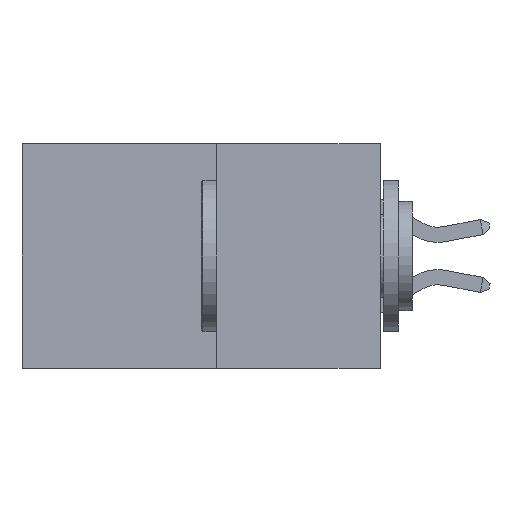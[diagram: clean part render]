
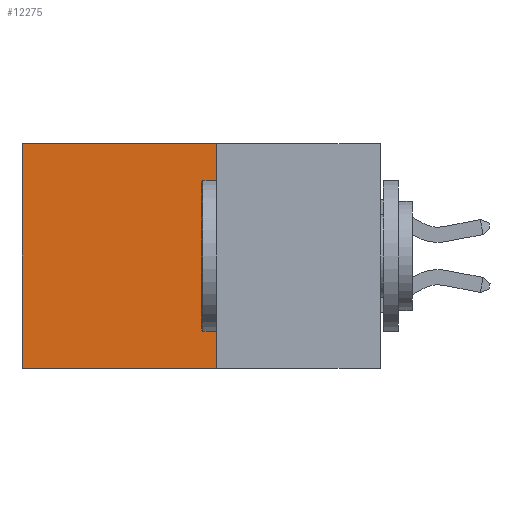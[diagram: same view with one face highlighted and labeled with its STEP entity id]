
A CAD part, left-side view. The second image highlights one B-rep face of the part: STEP entity #12275.
In plain terms, the highlighted planar face has unit normal (-1, 0, 0).
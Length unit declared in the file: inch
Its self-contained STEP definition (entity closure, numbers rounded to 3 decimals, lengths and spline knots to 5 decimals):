
#69 = ORIENTED_EDGE ( 'NONE', *, *, #7049, .F. ) ;
#188 = CARTESIAN_POINT ( 'NONE',  ( 0.277, 0.59, 0. ) ) ;
#551 = FACE_OUTER_BOUND ( 'NONE', #9237, .T. ) ;
#768 = DIRECTION ( 'NONE',  ( 0., 0., -1. ) ) ;
#949 = ORIENTED_EDGE ( 'NONE', *, *, #8611, .T. ) ;
#1112 = LINE ( 'NONE', #6383, #6055 ) ;
#1419 = DIRECTION ( 'NONE',  ( 0., 1., 0. ) ) ;
#1436 = CARTESIAN_POINT ( 'NONE',  ( 0.277, 0.27, 0. ) ) ;
#1829 = DIRECTION ( 'NONE',  ( 1., 0., 0. ) ) ;
#1876 = CARTESIAN_POINT ( 'NONE',  ( 0.277, 0.27, -0.37 ) ) ;
#2864 = PLANE ( 'NONE',  #3620 ) ;
#2878 = CARTESIAN_POINT ( 'NONE',  ( 0.277, 0.59, -0.37 ) ) ;
#2909 = VERTEX_POINT ( 'NONE', #2934 ) ;
#2934 = CARTESIAN_POINT ( 'NONE',  ( 0.277, 0.27, 0. ) ) ;
#3247 = EDGE_CURVE ( 'NONE', #4956, #11204, #1112, .T. ) ;
#3551 = VERTEX_POINT ( 'NONE', #188 ) ;
#3620 = AXIS2_PLACEMENT_3D ( 'NONE', #1876, #1829, #3857 ) ;
#3857 = DIRECTION ( 'NONE',  ( 0., 0., -1. ) ) ;
#4673 = ORIENTED_EDGE ( 'NONE', *, *, #12212, .T. ) ;
#4956 = VERTEX_POINT ( 'NONE', #9560 ) ;
#6055 = VECTOR ( 'NONE', #7109, 39.37008 ) ;
#6327 = LINE ( 'NONE', #10094, #11294 ) ;
#6383 = CARTESIAN_POINT ( 'NONE',  ( 0.277, 0.27, -0.37 ) ) ;
#7049 = EDGE_CURVE ( 'NONE', #2909, #4956, #6327, .T. ) ;
#7109 = DIRECTION ( 'NONE',  ( 0., 1., 0. ) ) ;
#7397 = ORIENTED_EDGE ( 'NONE', *, *, #3247, .F. ) ;
#8061 = VECTOR ( 'NONE', #1419, 39.37008 ) ;
#8611 = EDGE_CURVE ( 'NONE', #2909, #3551, #8692, .T. ) ;
#8633 = CARTESIAN_POINT ( 'NONE',  ( 0.277, 0.59, -0.37 ) ) ;
#8692 = LINE ( 'NONE', #1436, #8061 ) ;
#8767 = VECTOR ( 'NONE', #768, 39.37008 ) ;
#9237 = EDGE_LOOP ( 'NONE', ( #4673, #7397, #69, #949 ) ) ;
#9560 = CARTESIAN_POINT ( 'NONE',  ( 0.277, 0.27, -0.37 ) ) ;
#9989 = DIRECTION ( 'NONE',  ( 0., 0., -1. ) ) ;
#10094 = CARTESIAN_POINT ( 'NONE',  ( 0.277, 0.27, -0.37 ) ) ;
#11204 = VERTEX_POINT ( 'NONE', #2878 ) ;
#11294 = VECTOR ( 'NONE', #9989, 39.37008 ) ;
#11407 = LINE ( 'NONE', #8633, #8767 ) ;
#12212 = EDGE_CURVE ( 'NONE', #3551, #11204, #11407, .T. ) ;
#12275 = ADVANCED_FACE ( 'NONE', ( #551 ), #2864, .F. ) ;
